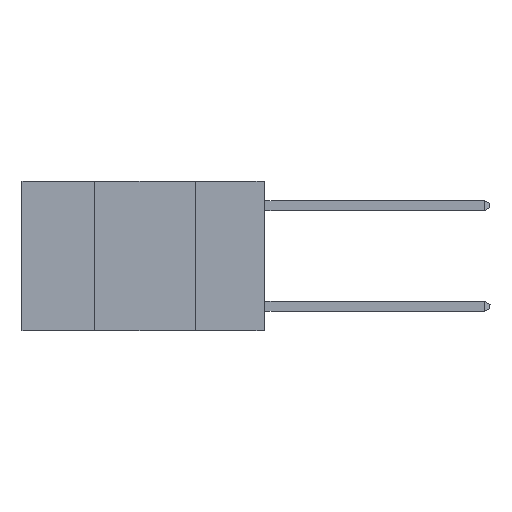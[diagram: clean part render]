
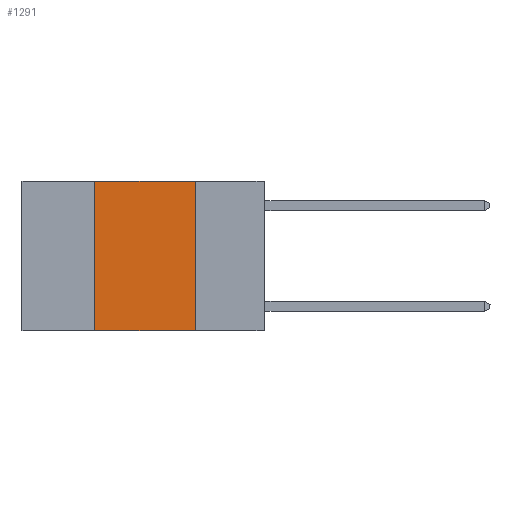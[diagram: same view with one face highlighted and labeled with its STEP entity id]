
A CAD part, left-side view. The second image highlights one B-rep face of the part: STEP entity #1291.
In plain terms, the highlighted planar face has unit normal (-1, 0, 0).
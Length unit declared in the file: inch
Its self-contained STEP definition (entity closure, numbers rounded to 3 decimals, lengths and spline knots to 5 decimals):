
#269 = LINE ( 'NONE', #6079, #9394 ) ;
#525 = ORIENTED_EDGE ( 'NONE', *, *, #17343, .F. ) ;
#1085 = CARTESIAN_POINT ( 'NONE',  ( 0., 0.6, 0. ) ) ;
#1263 = DIRECTION ( 'NONE',  ( 0., 0., 1. ) ) ;
#1291 = ADVANCED_FACE ( 'NONE', ( #17649 ), #14685, .F. ) ;
#2687 = EDGE_CURVE ( 'NONE', #12607, #11864, #13623, .T. ) ;
#3272 = VECTOR ( 'NONE', #1263, 39.37008 ) ;
#4041 = LINE ( 'NONE', #23213, #24123 ) ;
#4987 = DIRECTION ( 'NONE',  ( 0., 0., -1. ) ) ;
#6079 = CARTESIAN_POINT ( 'NONE',  ( 0., 0.17, 0. ) ) ;
#6689 = DIRECTION ( 'NONE',  ( 0., -1., 0. ) ) ;
#7477 = VERTEX_POINT ( 'NONE', #18580 ) ;
#9281 = ORIENTED_EDGE ( 'NONE', *, *, #14831, .T. ) ;
#9394 = VECTOR ( 'NONE', #23632, 39.37008 ) ;
#11864 = VERTEX_POINT ( 'NONE', #24792 ) ;
#11992 = CARTESIAN_POINT ( 'NONE',  ( 0., 0.17, 0. ) ) ;
#12607 = VERTEX_POINT ( 'NONE', #18631 ) ;
#13499 = DIRECTION ( 'NONE',  ( 0., -1., 0. ) ) ;
#13623 = LINE ( 'NONE', #14869, #3272 ) ;
#13842 = ORIENTED_EDGE ( 'NONE', *, *, #2687, .F. ) ;
#14685 = PLANE ( 'NONE',  #18887 ) ;
#14831 = EDGE_CURVE ( 'NONE', #12607, #7477, #4041, .T. ) ;
#14869 = CARTESIAN_POINT ( 'NONE',  ( 0., 0.42, 0. ) ) ;
#16574 = VECTOR ( 'NONE', #6689, 39.37008 ) ;
#16617 = EDGE_LOOP ( 'NONE', ( #525, #18434, #13842, #9281 ) ) ;
#16641 = DIRECTION ( 'NONE',  ( 1., 0., 0. ) ) ;
#17343 = EDGE_CURVE ( 'NONE', #20276, #7477, #269, .T. ) ;
#17649 = FACE_OUTER_BOUND ( 'NONE', #16617, .T. ) ;
#18434 = ORIENTED_EDGE ( 'NONE', *, *, #21169, .F. ) ;
#18580 = CARTESIAN_POINT ( 'NONE',  ( 0., 0.17, -0.37 ) ) ;
#18631 = CARTESIAN_POINT ( 'NONE',  ( 0., 0.42, -0.37 ) ) ;
#18887 = AXIS2_PLACEMENT_3D ( 'NONE', #1085, #16641, #4987 ) ;
#20276 = VERTEX_POINT ( 'NONE', #11992 ) ;
#21169 = EDGE_CURVE ( 'NONE', #11864, #20276, #22371, .T. ) ;
#22269 = CARTESIAN_POINT ( 'NONE',  ( 0., 0.6, 0. ) ) ;
#22371 = LINE ( 'NONE', #22269, #16574 ) ;
#23213 = CARTESIAN_POINT ( 'NONE',  ( 0., 0.6, -0.37 ) ) ;
#23632 = DIRECTION ( 'NONE',  ( 0., 0., -1. ) ) ;
#24123 = VECTOR ( 'NONE', #13499, 39.37008 ) ;
#24792 = CARTESIAN_POINT ( 'NONE',  ( 0., 0.42, 0. ) ) ;
